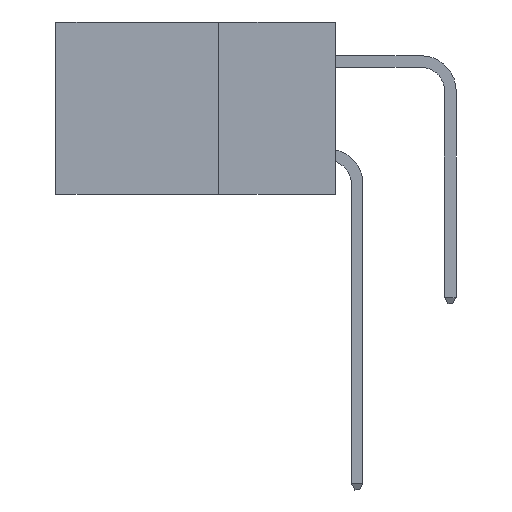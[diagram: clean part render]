
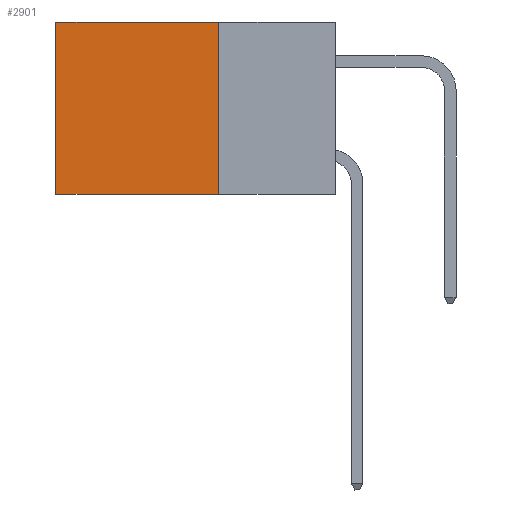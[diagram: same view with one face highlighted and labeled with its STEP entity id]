
A CAD part, left-side view. The second image highlights one B-rep face of the part: STEP entity #2901.
In plain terms, the highlighted planar face has unit normal (-1, 0, 0).
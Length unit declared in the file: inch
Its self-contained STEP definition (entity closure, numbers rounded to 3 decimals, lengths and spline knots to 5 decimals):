
#188 = VECTOR ( 'NONE', #688, 39.37008 ) ;
#269 = VERTEX_POINT ( 'NONE', #2961 ) ;
#328 = CARTESIAN_POINT ( 'NONE',  ( 0.2875, 0.6, -0.37 ) ) ;
#688 = DIRECTION ( 'NONE',  ( 0., 0., -1. ) ) ;
#1339 = DIRECTION ( 'NONE',  ( 0., 1., 0. ) ) ;
#1991 = DIRECTION ( 'NONE',  ( 0., 0., -1. ) ) ;
#2456 = VECTOR ( 'NONE', #12341, 39.37008 ) ;
#2567 = ORIENTED_EDGE ( 'NONE', *, *, #3308, .T. ) ;
#2901 = ADVANCED_FACE ( 'NONE', ( #11448 ), #7972, .F. ) ;
#2961 = CARTESIAN_POINT ( 'NONE',  ( 0.2875, 0.25, -0.37 ) ) ;
#3208 = CARTESIAN_POINT ( 'NONE',  ( 0.2875, 0.25, 0. ) ) ;
#3308 = EDGE_CURVE ( 'NONE', #14806, #12717, #12808, .T. ) ;
#3397 = CARTESIAN_POINT ( 'NONE',  ( 0.2875, 0.25, 0. ) ) ;
#3455 = ORIENTED_EDGE ( 'NONE', *, *, #3620, .F. ) ;
#3480 = DIRECTION ( 'NONE',  ( 0., 0., -1. ) ) ;
#3620 = EDGE_CURVE ( 'NONE', #269, #5862, #10065, .T. ) ;
#4541 = VECTOR ( 'NONE', #1991, 39.37008 ) ;
#4875 = ORIENTED_EDGE ( 'NONE', *, *, #13181, .F. ) ;
#5862 = VERTEX_POINT ( 'NONE', #328 ) ;
#7716 = CARTESIAN_POINT ( 'NONE',  ( 0.2875, 0.25, -0.37 ) ) ;
#7972 = PLANE ( 'NONE',  #14656 ) ;
#8296 = EDGE_LOOP ( 'NONE', ( #13453, #3455, #4875, #2567 ) ) ;
#8760 = LINE ( 'NONE', #3208, #4541 ) ;
#9187 = DIRECTION ( 'NONE',  ( 1., 0., 0. ) ) ;
#9530 = CARTESIAN_POINT ( 'NONE',  ( 0.2875, 0.25, 0. ) ) ;
#10065 = LINE ( 'NONE', #7716, #2456 ) ;
#10805 = VECTOR ( 'NONE', #1339, 39.37008 ) ;
#11448 = FACE_OUTER_BOUND ( 'NONE', #8296, .T. ) ;
#12079 = LINE ( 'NONE', #14336, #188 ) ;
#12341 = DIRECTION ( 'NONE',  ( 0., 1., 0. ) ) ;
#12717 = VERTEX_POINT ( 'NONE', #14261 ) ;
#12780 = EDGE_CURVE ( 'NONE', #12717, #5862, #12079, .T. ) ;
#12808 = LINE ( 'NONE', #3397, #10805 ) ;
#12823 = CARTESIAN_POINT ( 'NONE',  ( 0.2875, 0.25, 0. ) ) ;
#13181 = EDGE_CURVE ( 'NONE', #14806, #269, #8760, .T. ) ;
#13453 = ORIENTED_EDGE ( 'NONE', *, *, #12780, .T. ) ;
#14261 = CARTESIAN_POINT ( 'NONE',  ( 0.2875, 0.6, 0. ) ) ;
#14336 = CARTESIAN_POINT ( 'NONE',  ( 0.2875, 0.6, 0. ) ) ;
#14656 = AXIS2_PLACEMENT_3D ( 'NONE', #12823, #9187, #3480 ) ;
#14806 = VERTEX_POINT ( 'NONE', #9530 ) ;
